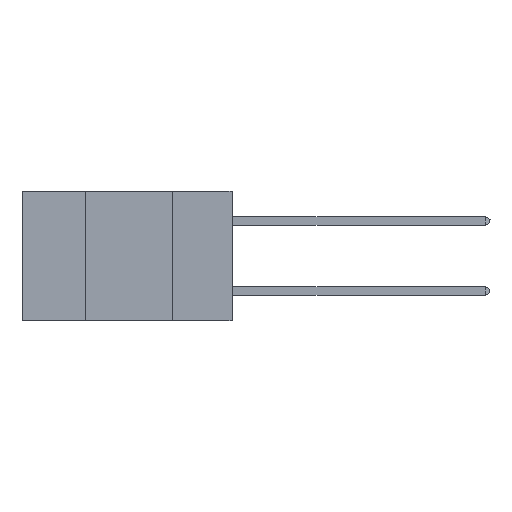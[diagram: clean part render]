
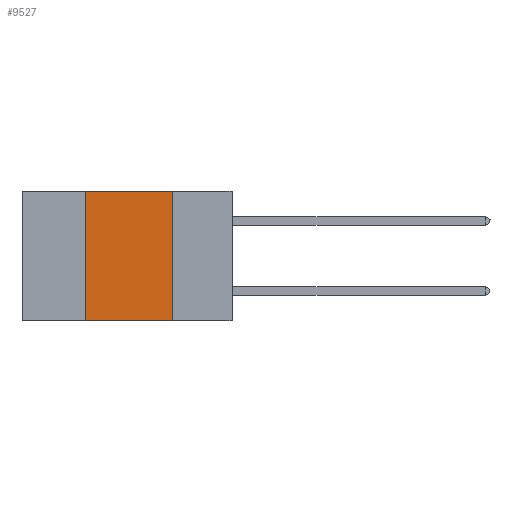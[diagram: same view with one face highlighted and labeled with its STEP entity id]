
A CAD part, left-side view. The second image highlights one B-rep face of the part: STEP entity #9527.
In plain terms, the highlighted planar face has unit normal (-1, 0, 0).
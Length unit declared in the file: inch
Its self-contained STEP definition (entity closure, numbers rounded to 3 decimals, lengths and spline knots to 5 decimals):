
#282 = VERTEX_POINT ( 'NONE', #26373 ) ;
#1496 = ORIENTED_EDGE ( 'NONE', *, *, #37183, .T. ) ;
#2940 = LINE ( 'NONE', #16676, #13634 ) ;
#3425 = LINE ( 'NONE', #17164, #38441 ) ;
#3688 = DIRECTION ( 'NONE',  ( 0., -1., 0. ) ) ;
#5831 = VERTEX_POINT ( 'NONE', #24087 ) ;
#6404 = CARTESIAN_POINT ( 'NONE',  ( 0., 0.6, -0.37 ) ) ;
#8548 = FACE_OUTER_BOUND ( 'NONE', #11579, .T. ) ;
#9527 = ADVANCED_FACE ( 'NONE', ( #8548 ), #36100, .F. ) ;
#11579 = EDGE_LOOP ( 'NONE', ( #41092, #40889, #18419, #1496 ) ) ;
#13634 = VECTOR ( 'NONE', #27915, 39.37008 ) ;
#13789 = DIRECTION ( 'NONE',  ( 0., 0., -1. ) ) ;
#15513 = CARTESIAN_POINT ( 'NONE',  ( 0., 0.6, 0. ) ) ;
#16676 = CARTESIAN_POINT ( 'NONE',  ( 0., 0.42, 0. ) ) ;
#17164 = CARTESIAN_POINT ( 'NONE',  ( 0., 0.17, 0. ) ) ;
#18014 = AXIS2_PLACEMENT_3D ( 'NONE', #15513, #43095, #22743 ) ;
#18419 = ORIENTED_EDGE ( 'NONE', *, *, #24722, .F. ) ;
#18740 = VECTOR ( 'NONE', #27006, 39.37008 ) ;
#20327 = VERTEX_POINT ( 'NONE', #34643 ) ;
#22743 = DIRECTION ( 'NONE',  ( 0., 0., -1. ) ) ;
#23542 = LINE ( 'NONE', #6404, #25722 ) ;
#24087 = CARTESIAN_POINT ( 'NONE',  ( 0., 0.42, 0. ) ) ;
#24722 = EDGE_CURVE ( 'NONE', #20327, #5831, #2940, .T. ) ;
#25722 = VECTOR ( 'NONE', #3688, 39.37008 ) ;
#26373 = CARTESIAN_POINT ( 'NONE',  ( 0., 0.17, 0. ) ) ;
#26392 = EDGE_CURVE ( 'NONE', #5831, #282, #27451, .T. ) ;
#27006 = DIRECTION ( 'NONE',  ( 0., -1., 0. ) ) ;
#27451 = LINE ( 'NONE', #38079, #18740 ) ;
#27915 = DIRECTION ( 'NONE',  ( 0., 0., 1. ) ) ;
#32739 = EDGE_CURVE ( 'NONE', #282, #33579, #3425, .T. ) ;
#33579 = VERTEX_POINT ( 'NONE', #33977 ) ;
#33977 = CARTESIAN_POINT ( 'NONE',  ( 0., 0.17, -0.37 ) ) ;
#34643 = CARTESIAN_POINT ( 'NONE',  ( 0., 0.42, -0.37 ) ) ;
#36100 = PLANE ( 'NONE',  #18014 ) ;
#37183 = EDGE_CURVE ( 'NONE', #20327, #33579, #23542, .T. ) ;
#38079 = CARTESIAN_POINT ( 'NONE',  ( 0., 0.6, 0. ) ) ;
#38441 = VECTOR ( 'NONE', #13789, 39.37008 ) ;
#40889 = ORIENTED_EDGE ( 'NONE', *, *, #26392, .F. ) ;
#41092 = ORIENTED_EDGE ( 'NONE', *, *, #32739, .F. ) ;
#43095 = DIRECTION ( 'NONE',  ( 1., 0., 0. ) ) ;
